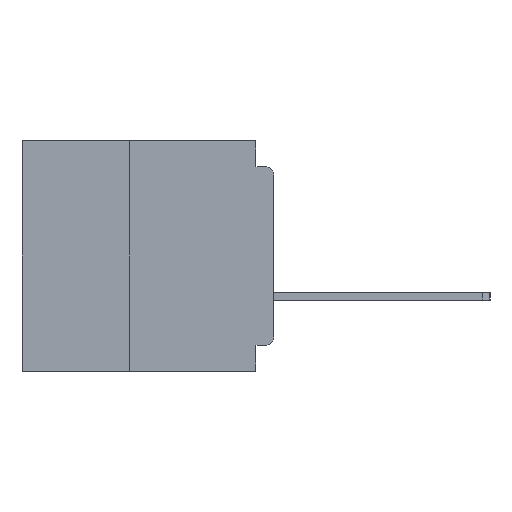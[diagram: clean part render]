
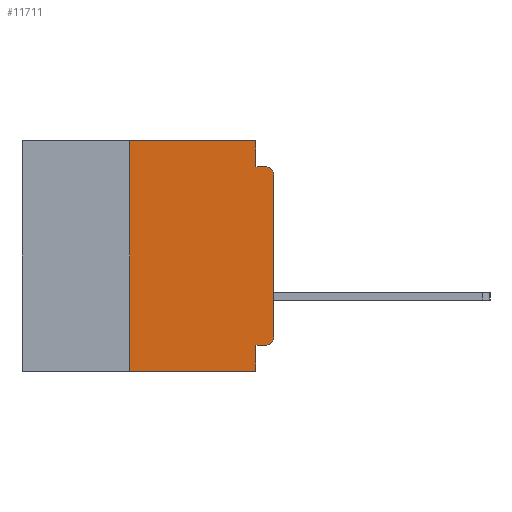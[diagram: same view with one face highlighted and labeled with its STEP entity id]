
A CAD part, left-side view. The second image highlights one B-rep face of the part: STEP entity #11711.
In plain terms, the highlighted planar face has unit normal (-1, 0, 0).
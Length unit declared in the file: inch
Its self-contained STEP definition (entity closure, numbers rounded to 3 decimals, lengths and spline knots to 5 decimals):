
#145 = ORIENTED_EDGE ( 'NONE', *, *, #6568, .F. ) ;
#803 = CARTESIAN_POINT ( 'NONE',  ( 0., 0.031, -0.045 ) ) ;
#2644 = LINE ( 'NONE', #15900, #49797 ) ;
#2861 = CARTESIAN_POINT ( 'NONE',  ( 0., 0.031, 0. ) ) ;
#2947 = CARTESIAN_POINT ( 'NONE',  ( 0., 0.015, -0.06 ) ) ;
#3202 = DIRECTION ( 'NONE',  ( 0., 0., -1. ) ) ;
#3733 = EDGE_CURVE ( 'NONE', #54923, #36226, #29543, .T. ) ;
#4300 = EDGE_CURVE ( 'NONE', #54923, #47414, #58094, .T. ) ;
#5012 = CARTESIAN_POINT ( 'NONE',  ( 0., 0., -0.045 ) ) ;
#5104 = CARTESIAN_POINT ( 'NONE',  ( 0., 0.015, -0.045 ) ) ;
#5940 = VECTOR ( 'NONE', #56667, 39.37008 ) ;
#6043 = VERTEX_POINT ( 'NONE', #22547 ) ;
#6568 = EDGE_CURVE ( 'NONE', #6043, #61049, #7077, .T. ) ;
#6874 = VERTEX_POINT ( 'NONE', #5104 ) ;
#7077 = LINE ( 'NONE', #2861, #21127 ) ;
#7712 = DIRECTION ( 'NONE',  ( 0., 0., -1. ) ) ;
#10441 = CARTESIAN_POINT ( 'NONE',  ( 0., 0.437, -0.4 ) ) ;
#11689 = FACE_OUTER_BOUND ( 'NONE', #32713, .T. ) ;
#11711 = ADVANCED_FACE ( 'NONE', ( #11689 ), #44338, .F. ) ;
#12684 = CARTESIAN_POINT ( 'NONE',  ( 0., 0.437, 0. ) ) ;
#12837 = EDGE_CURVE ( 'NONE', #35043, #58830, #51771, .T. ) ;
#12913 = VECTOR ( 'NONE', #25677, 39.37008 ) ;
#13184 = CARTESIAN_POINT ( 'NONE',  ( 0., 0.015, -0.355 ) ) ;
#14104 = EDGE_CURVE ( 'NONE', #61049, #6874, #43559, .T. ) ;
#15900 = CARTESIAN_POINT ( 'NONE',  ( 0., 0., 0. ) ) ;
#16375 = CARTESIAN_POINT ( 'NONE',  ( 0., 0., -0.34 ) ) ;
#16668 = VECTOR ( 'NONE', #52775, 39.37008 ) ;
#17014 = VECTOR ( 'NONE', #31345, 39.37008 ) ;
#17025 = CARTESIAN_POINT ( 'NONE',  ( 0., 0., -0.06 ) ) ;
#17435 = DIRECTION ( 'NONE',  ( 0., -1., 0. ) ) ;
#18545 = EDGE_CURVE ( 'NONE', #48144, #6043, #24644, .T. ) ;
#19922 = CARTESIAN_POINT ( 'NONE',  ( 0., 0.031, -0.4 ) ) ;
#20086 = VERTEX_POINT ( 'NONE', #17025 ) ;
#20887 = DIRECTION ( 'NONE',  ( 1., 0., 0. ) ) ;
#21127 = VECTOR ( 'NONE', #40607, 39.37008 ) ;
#22234 = AXIS2_PLACEMENT_3D ( 'NONE', #49035, #20887, #53754 ) ;
#22547 = CARTESIAN_POINT ( 'NONE',  ( 0., 0.031, 0. ) ) ;
#24644 = LINE ( 'NONE', #12684, #35667 ) ;
#25234 = CARTESIAN_POINT ( 'NONE',  ( 0., 0.031, -0.4 ) ) ;
#25677 = DIRECTION ( 'NONE',  ( 0., 0., 1. ) ) ;
#27161 = EDGE_CURVE ( 'NONE', #47414, #20086, #2644, .T. ) ;
#29211 = LINE ( 'NONE', #19922, #16668 ) ;
#29543 = LINE ( 'NONE', #50025, #17014 ) ;
#30912 = AXIS2_PLACEMENT_3D ( 'NONE', #2947, #35931, #7712 ) ;
#31345 = DIRECTION ( 'NONE',  ( 0., 1., 0. ) ) ;
#31467 = DIRECTION ( 'NONE',  ( -1., 0., 0. ) ) ;
#32457 = ORIENTED_EDGE ( 'NONE', *, *, #4300, .T. ) ;
#32713 = EDGE_LOOP ( 'NONE', ( #46708, #50455, #55728, #145, #50447, #35194, #49843, #44132, #36403, #32457 ) ) ;
#33438 = CARTESIAN_POINT ( 'NONE',  ( 0., 0.25, 0. ) ) ;
#34796 = DIRECTION ( 'NONE',  ( 0., 0., 1. ) ) ;
#35043 = VERTEX_POINT ( 'NONE', #35088 ) ;
#35088 = CARTESIAN_POINT ( 'NONE',  ( 0., 0.25, -0.4 ) ) ;
#35194 = ORIENTED_EDGE ( 'NONE', *, *, #45030, .F. ) ;
#35667 = VECTOR ( 'NONE', #17435, 39.37008 ) ;
#35931 = DIRECTION ( 'NONE',  ( -1., 0., 0. ) ) ;
#36226 = VERTEX_POINT ( 'NONE', #41732 ) ;
#36403 = ORIENTED_EDGE ( 'NONE', *, *, #3733, .F. ) ;
#38382 = EDGE_CURVE ( 'NONE', #20086, #6874, #58108, .T. ) ;
#39311 = VECTOR ( 'NONE', #52796, 39.37008 ) ;
#40607 = DIRECTION ( 'NONE',  ( 0., 0., -1. ) ) ;
#41732 = CARTESIAN_POINT ( 'NONE',  ( 0., 0.031, -0.355 ) ) ;
#43559 = LINE ( 'NONE', #5012, #5940 ) ;
#44132 = ORIENTED_EDGE ( 'NONE', *, *, #55184, .F. ) ;
#44338 = PLANE ( 'NONE',  #22234 ) ;
#44397 = CARTESIAN_POINT ( 'NONE',  ( 0., 0.25, -0.4 ) ) ;
#45030 = EDGE_CURVE ( 'NONE', #35043, #48144, #51880, .T. ) ;
#46708 = ORIENTED_EDGE ( 'NONE', *, *, #27161, .T. ) ;
#47414 = VERTEX_POINT ( 'NONE', #16375 ) ;
#48144 = VERTEX_POINT ( 'NONE', #33438 ) ;
#49035 = CARTESIAN_POINT ( 'NONE',  ( 0., 0.437, 0. ) ) ;
#49797 = VECTOR ( 'NONE', #34796, 39.37008 ) ;
#49843 = ORIENTED_EDGE ( 'NONE', *, *, #12837, .T. ) ;
#50025 = CARTESIAN_POINT ( 'NONE',  ( 0., 0., -0.355 ) ) ;
#50447 = ORIENTED_EDGE ( 'NONE', *, *, #18545, .F. ) ;
#50455 = ORIENTED_EDGE ( 'NONE', *, *, #38382, .T. ) ;
#51771 = LINE ( 'NONE', #10441, #39311 ) ;
#51880 = LINE ( 'NONE', #44397, #12913 ) ;
#52775 = DIRECTION ( 'NONE',  ( 0., 0., -1. ) ) ;
#52796 = DIRECTION ( 'NONE',  ( 0., -1., 0. ) ) ;
#53754 = DIRECTION ( 'NONE',  ( 0., 0., -1. ) ) ;
#53818 = AXIS2_PLACEMENT_3D ( 'NONE', #59602, #31467, #3202 ) ;
#54923 = VERTEX_POINT ( 'NONE', #13184 ) ;
#55184 = EDGE_CURVE ( 'NONE', #36226, #58830, #29211, .T. ) ;
#55728 = ORIENTED_EDGE ( 'NONE', *, *, #14104, .F. ) ;
#56667 = DIRECTION ( 'NONE',  ( 0., -1., 0. ) ) ;
#58094 = CIRCLE ( 'NONE', #53818, 0.015 ) ;
#58108 = CIRCLE ( 'NONE', #30912, 0.015 ) ;
#58830 = VERTEX_POINT ( 'NONE', #25234 ) ;
#59602 = CARTESIAN_POINT ( 'NONE',  ( 0., 0.015, -0.34 ) ) ;
#61049 = VERTEX_POINT ( 'NONE', #803 ) ;
